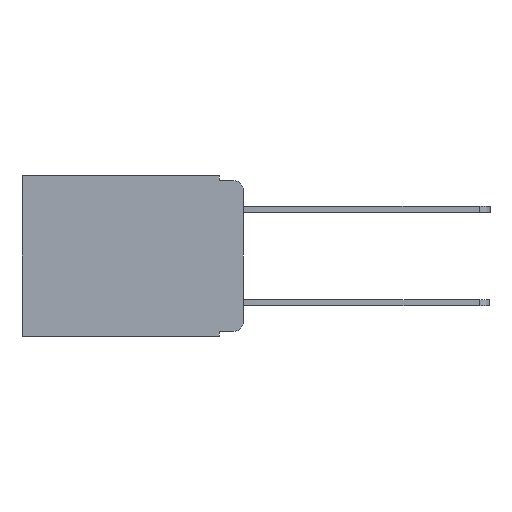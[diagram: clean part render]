
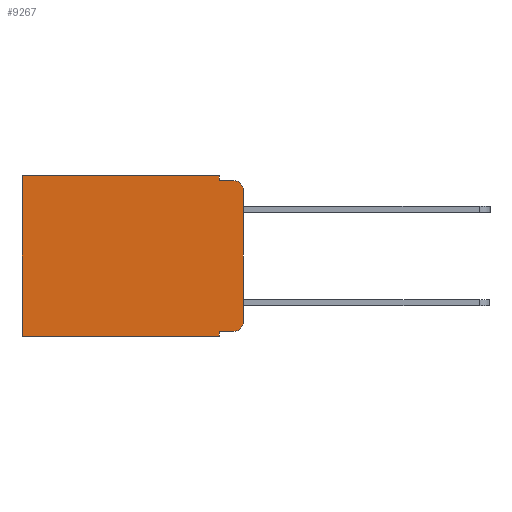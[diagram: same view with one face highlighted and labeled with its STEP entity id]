
A CAD part, left-side view. The second image highlights one B-rep face of the part: STEP entity #9267.
In plain terms, the highlighted planar face has unit normal (-1, 0, 0).
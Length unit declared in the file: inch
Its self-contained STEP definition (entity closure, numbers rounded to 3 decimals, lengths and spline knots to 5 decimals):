
#186 = CIRCLE ( 'NONE', #10538, 0.02 ) ;
#296 = ORIENTED_EDGE ( 'NONE', *, *, #7115, .F. ) ;
#503 = CARTESIAN_POINT ( 'NONE',  ( 0.298, 0.473, 0. ) ) ;
#801 = CARTESIAN_POINT ( 'NONE',  ( 0.298, 0.473, 0. ) ) ;
#875 = ORIENTED_EDGE ( 'NONE', *, *, #5936, .T. ) ;
#1009 = DIRECTION ( 'NONE',  ( 0., 0., -1. ) ) ;
#1210 = ORIENTED_EDGE ( 'NONE', *, *, #7390, .T. ) ;
#1307 = ORIENTED_EDGE ( 'NONE', *, *, #9402, .F. ) ;
#1987 = CARTESIAN_POINT ( 'NONE',  ( 0.298, 0., 0. ) ) ;
#2297 = LINE ( 'NONE', #10210, #6658 ) ;
#2354 = CARTESIAN_POINT ( 'NONE',  ( 0.298, 0.051, -0.01 ) ) ;
#2775 = CARTESIAN_POINT ( 'NONE',  ( 0.298, 0.051, -0.333 ) ) ;
#3094 = DIRECTION ( 'NONE',  ( 1., 0., 0. ) ) ;
#3158 = DIRECTION ( 'NONE',  ( -1., 0., 0. ) ) ;
#3266 = CARTESIAN_POINT ( 'NONE',  ( 0.298, 0., -0.313 ) ) ;
#3458 = DIRECTION ( 'NONE',  ( 0., 0., -1. ) ) ;
#3613 = VERTEX_POINT ( 'NONE', #3266 ) ;
#3850 = DIRECTION ( 'NONE',  ( 0., 0., -1. ) ) ;
#3857 = LINE ( 'NONE', #5442, #10657 ) ;
#3894 = ORIENTED_EDGE ( 'NONE', *, *, #8308, .T. ) ;
#4186 = AXIS2_PLACEMENT_3D ( 'NONE', #8317, #3094, #9140 ) ;
#4218 = EDGE_CURVE ( 'NONE', #6432, #7605, #2297, .T. ) ;
#4262 = VERTEX_POINT ( 'NONE', #2354 ) ;
#4278 = CARTESIAN_POINT ( 'NONE',  ( 0.298, 0.473, -0.343 ) ) ;
#4305 = ORIENTED_EDGE ( 'NONE', *, *, #4218, .F. ) ;
#4553 = VECTOR ( 'NONE', #8905, 39.37008 ) ;
#4788 = EDGE_CURVE ( 'NONE', #7387, #7097, #9988, .T. ) ;
#4864 = LINE ( 'NONE', #5391, #6621 ) ;
#5174 = CARTESIAN_POINT ( 'NONE',  ( 0.298, 0.02, -0.03 ) ) ;
#5391 = CARTESIAN_POINT ( 'NONE',  ( 0.298, 0.051, 0. ) ) ;
#5438 = VECTOR ( 'NONE', #8871, 39.37008 ) ;
#5442 = CARTESIAN_POINT ( 'NONE',  ( 0.298, 0., 0. ) ) ;
#5523 = VECTOR ( 'NONE', #10105, 39.37008 ) ;
#5909 = CARTESIAN_POINT ( 'NONE',  ( 0.298, 0.02, -0.333 ) ) ;
#5917 = DIRECTION ( 'NONE',  ( 0., -1., 0. ) ) ;
#5936 = EDGE_CURVE ( 'NONE', #7097, #3613, #186, .T. ) ;
#5967 = CARTESIAN_POINT ( 'NONE',  ( 0.298, 0.051, 0. ) ) ;
#6036 = CARTESIAN_POINT ( 'NONE',  ( 0.298, 0., -0.03 ) ) ;
#6142 = CARTESIAN_POINT ( 'NONE',  ( 0.298, 0.02, -0.01 ) ) ;
#6318 = ORIENTED_EDGE ( 'NONE', *, *, #7710, .T. ) ;
#6330 = CARTESIAN_POINT ( 'NONE',  ( 0.298, 0.051, -0.343 ) ) ;
#6403 = CARTESIAN_POINT ( 'NONE',  ( 0.298, 0.02, -0.313 ) ) ;
#6432 = VERTEX_POINT ( 'NONE', #6330 ) ;
#6528 = EDGE_CURVE ( 'NONE', #7769, #4262, #4864, .T. ) ;
#6538 = PLANE ( 'NONE',  #4186 ) ;
#6621 = VECTOR ( 'NONE', #8001, 39.37008 ) ;
#6658 = VECTOR ( 'NONE', #10299, 39.37008 ) ;
#6874 = LINE ( 'NONE', #1987, #4553 ) ;
#6951 = ORIENTED_EDGE ( 'NONE', *, *, #11043, .F. ) ;
#7097 = VERTEX_POINT ( 'NONE', #5909 ) ;
#7115 = EDGE_CURVE ( 'NONE', #7387, #6432, #7843, .T. ) ;
#7313 = FACE_OUTER_BOUND ( 'NONE', #9927, .T. ) ;
#7387 = VERTEX_POINT ( 'NONE', #2775 ) ;
#7390 = EDGE_CURVE ( 'NONE', #7769, #9965, #6874, .T. ) ;
#7605 = VERTEX_POINT ( 'NONE', #4278 ) ;
#7619 = AXIS2_PLACEMENT_3D ( 'NONE', #5174, #11123, #3458 ) ;
#7710 = EDGE_CURVE ( 'NONE', #8904, #10680, #8520, .T. ) ;
#7769 = VERTEX_POINT ( 'NONE', #10132 ) ;
#7843 = LINE ( 'NONE', #5967, #5523 ) ;
#8001 = DIRECTION ( 'NONE',  ( 0., 0., -1. ) ) ;
#8034 = CARTESIAN_POINT ( 'NONE',  ( 0.298, 0.051, -0.333 ) ) ;
#8276 = VECTOR ( 'NONE', #5917, 39.37008 ) ;
#8308 = EDGE_CURVE ( 'NONE', #9965, #7605, #11056, .T. ) ;
#8317 = CARTESIAN_POINT ( 'NONE',  ( 0.298, 0., 0. ) ) ;
#8520 = CIRCLE ( 'NONE', #7619, 0.02 ) ;
#8871 = DIRECTION ( 'NONE',  ( 0., -1., 0. ) ) ;
#8878 = VECTOR ( 'NONE', #10392, 39.37008 ) ;
#8904 = VERTEX_POINT ( 'NONE', #6036 ) ;
#8905 = DIRECTION ( 'NONE',  ( 0., 1., 0. ) ) ;
#9140 = DIRECTION ( 'NONE',  ( 0., 0., -1. ) ) ;
#9267 = ADVANCED_FACE ( 'NONE', ( #7313 ), #6538, .F. ) ;
#9402 = EDGE_CURVE ( 'NONE', #4262, #10680, #10188, .T. ) ;
#9750 = ORIENTED_EDGE ( 'NONE', *, *, #4788, .T. ) ;
#9927 = EDGE_LOOP ( 'NONE', ( #6951, #6318, #1307, #10536, #1210, #3894, #4305, #296, #9750, #875 ) ) ;
#9965 = VERTEX_POINT ( 'NONE', #503 ) ;
#9988 = LINE ( 'NONE', #8034, #5438 ) ;
#10105 = DIRECTION ( 'NONE',  ( 0., 0., -1. ) ) ;
#10132 = CARTESIAN_POINT ( 'NONE',  ( 0.298, 0.051, 0. ) ) ;
#10188 = LINE ( 'NONE', #10995, #8276 ) ;
#10210 = CARTESIAN_POINT ( 'NONE',  ( 0.298, 0., -0.343 ) ) ;
#10299 = DIRECTION ( 'NONE',  ( 0., 1., 0. ) ) ;
#10392 = DIRECTION ( 'NONE',  ( 0., 0., -1. ) ) ;
#10536 = ORIENTED_EDGE ( 'NONE', *, *, #6528, .F. ) ;
#10538 = AXIS2_PLACEMENT_3D ( 'NONE', #6403, #3158, #3850 ) ;
#10657 = VECTOR ( 'NONE', #1009, 39.37008 ) ;
#10680 = VERTEX_POINT ( 'NONE', #6142 ) ;
#10995 = CARTESIAN_POINT ( 'NONE',  ( 0.298, 0.051, -0.01 ) ) ;
#11043 = EDGE_CURVE ( 'NONE', #8904, #3613, #3857, .T. ) ;
#11056 = LINE ( 'NONE', #801, #8878 ) ;
#11123 = DIRECTION ( 'NONE',  ( -1., 0., 0. ) ) ;
